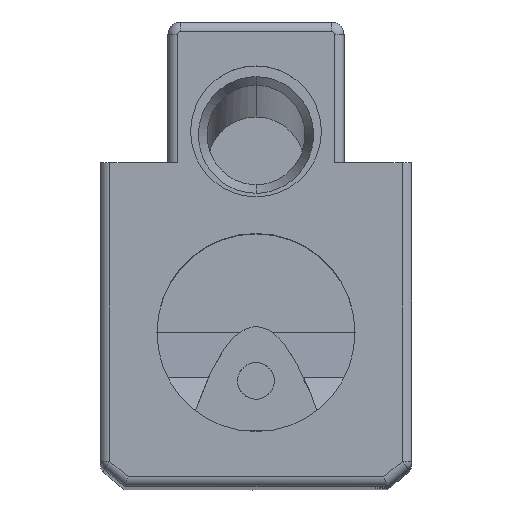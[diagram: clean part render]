
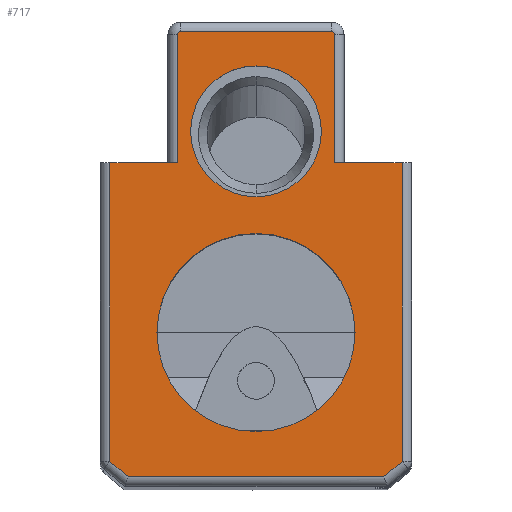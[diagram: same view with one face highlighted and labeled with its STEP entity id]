
A CAD part, top view. The second image highlights one B-rep face of the part: STEP entity #717.
In plain terms, the highlighted planar face has unit normal (0, 0, 1).
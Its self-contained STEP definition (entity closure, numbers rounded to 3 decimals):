
#1 = CARTESIAN_POINT ( 'NONE',  ( 8.1, -0.65, 0. ) ) ;
#50 = EDGE_LOOP ( 'NONE', ( #1934, #164 ) ) ;
#64 = VERTEX_POINT ( 'NONE', #5899 ) ;
#115 = AXIS2_PLACEMENT_3D ( 'NONE', #4630, #5019, #1920 ) ;
#150 = VERTEX_POINT ( 'NONE', #1952 ) ;
#164 = ORIENTED_EDGE ( 'NONE', *, *, #4117, .T. ) ;
#181 = DIRECTION ( 'NONE',  ( 1., 0., 0. ) ) ;
#234 = CARTESIAN_POINT ( 'NONE',  ( -6.2, 23.75, 0. ) ) ;
#284 = LINE ( 'NONE', #801, #3854 ) ;
#332 = EDGE_CURVE ( 'NONE', #5926, #869, #5600, .T. ) ;
#378 = ORIENTED_EDGE ( 'NONE', *, *, #2309, .F. ) ;
#432 = ORIENTED_EDGE ( 'NONE', *, *, #545, .T. ) ;
#531 = DIRECTION ( 'NONE',  ( 0., -1., 0. ) ) ;
#545 = EDGE_CURVE ( 'NONE', #1265, #2076, #2159, .T. ) ;
#591 = DIRECTION ( 'NONE',  ( 1., 0., 0. ) ) ;
#624 = CARTESIAN_POINT ( 'NONE',  ( 6.4, 23.75, 0. ) ) ;
#664 = CARTESIAN_POINT ( 'NONE',  ( 0., -0.65, 0. ) ) ;
#717 = ADVANCED_FACE ( 'NONE', ( #4224, #2316, #2632 ), #4130, .F. ) ;
#801 = CARTESIAN_POINT ( 'NONE',  ( -12.75, 13.25, 0. ) ) ;
#869 = VERTEX_POINT ( 'NONE', #1933 ) ;
#882 = VERTEX_POINT ( 'NONE', #3856 ) ;
#899 = DIRECTION ( 'NONE',  ( -0.766, -0.643, 0. ) ) ;
#955 = VERTEX_POINT ( 'NONE', #1 ) ;
#968 = ORIENTED_EDGE ( 'NONE', *, *, #332, .F. ) ;
#1054 = DIRECTION ( 'NONE',  ( -1., 0., 0. ) ) ;
#1068 = EDGE_CURVE ( 'NONE', #2082, #5395, #1801, .T. ) ;
#1101 = CARTESIAN_POINT ( 'NONE',  ( 5.35, 15.8, 0. ) ) ;
#1108 = DIRECTION ( 'NONE',  ( -1., 0., 0. ) ) ;
#1265 = VERTEX_POINT ( 'NONE', #624 ) ;
#1324 = ORIENTED_EDGE ( 'NONE', *, *, #4076, .T. ) ;
#1344 = EDGE_CURVE ( 'NONE', #5395, #2082, #5387, .T. ) ;
#1346 = EDGE_CURVE ( 'NONE', #150, #6261, #4244, .T. ) ;
#1401 = LINE ( 'NONE', #3632, #1552 ) ;
#1410 = AXIS2_PLACEMENT_3D ( 'NONE', #1907, #3327, #591 ) ;
#1411 = DIRECTION ( 'NONE',  ( 0., 0., -1. ) ) ;
#1472 = DIRECTION ( 'NONE',  ( 0., 0., -1. ) ) ;
#1508 = DIRECTION ( 'NONE',  ( 0., -1., 0. ) ) ;
#1552 = VECTOR ( 'NONE', #899, 1000. ) ;
#1577 = DIRECTION ( 'NONE',  ( -1., 0., 0. ) ) ;
#1602 = CARTESIAN_POINT ( 'NONE',  ( 11.95, -11.199, 0. ) ) ;
#1708 = AXIS2_PLACEMENT_3D ( 'NONE', #664, #1472, #1577 ) ;
#1737 = CARTESIAN_POINT ( 'NONE',  ( 10.459, -12.45, 0. ) ) ;
#1741 = ORIENTED_EDGE ( 'NONE', *, *, #3495, .T. ) ;
#1768 = AXIS2_PLACEMENT_3D ( 'NONE', #2861, #2649, #6206 ) ;
#1801 = CIRCLE ( 'NONE', #1410, 5.35 ) ;
#1907 = CARTESIAN_POINT ( 'NONE',  ( 0., 15.8, 0. ) ) ;
#1920 = DIRECTION ( 'NONE',  ( -1., 0., 0. ) ) ;
#1933 = CARTESIAN_POINT ( 'NONE',  ( -11.95, -11.199, 0. ) ) ;
#1934 = ORIENTED_EDGE ( 'NONE', *, *, #4635, .T. ) ;
#1951 = EDGE_CURVE ( 'NONE', #882, #150, #3329, .T. ) ;
#1952 = CARTESIAN_POINT ( 'NONE',  ( -6.4, 23.75, 0. ) ) ;
#1957 = EDGE_CURVE ( 'NONE', #869, #2942, #2252, .T. ) ;
#2065 = LINE ( 'NONE', #4367, #2939 ) ;
#2076 = VERTEX_POINT ( 'NONE', #4369 ) ;
#2082 = VERTEX_POINT ( 'NONE', #4871 ) ;
#2098 = VECTOR ( 'NONE', #4193, 1000. ) ;
#2135 = CARTESIAN_POINT ( 'NONE',  ( -10.459, -12.45, 0. ) ) ;
#2159 = CIRCLE ( 'NONE', #115, 0.2 ) ;
#2170 = CARTESIAN_POINT ( 'NONE',  ( -11.95, 13.25, 0. ) ) ;
#2176 = EDGE_LOOP ( 'NONE', ( #2567, #5139, #5936, #968, #3387, #4484, #378, #5836, #1324, #432, #1741, #4733 ) ) ;
#2223 = VERTEX_POINT ( 'NONE', #1602 ) ;
#2252 = LINE ( 'NONE', #5588, #5330 ) ;
#2261 = CARTESIAN_POINT ( 'NONE',  ( -6.2, 23.95, 0. ) ) ;
#2309 = EDGE_CURVE ( 'NONE', #4517, #2223, #3640, .T. ) ;
#2316 = FACE_OUTER_BOUND ( 'NONE', #2176, .T. ) ;
#2438 = VERTEX_POINT ( 'NONE', #1737 ) ;
#2483 = LINE ( 'NONE', #2261, #2767 ) ;
#2567 = ORIENTED_EDGE ( 'NONE', *, *, #1346, .T. ) ;
#2632 = FACE_BOUND ( 'NONE', #3348, .T. ) ;
#2649 = DIRECTION ( 'NONE',  ( 0., 0., 1. ) ) ;
#2767 = VECTOR ( 'NONE', #5596, 1000. ) ;
#2789 = VECTOR ( 'NONE', #1508, 1000. ) ;
#2861 = CARTESIAN_POINT ( 'NONE',  ( 0., 15.8, 0. ) ) ;
#2939 = VECTOR ( 'NONE', #4957, 1000. ) ;
#2942 = VERTEX_POINT ( 'NONE', #2170 ) ;
#3031 = EDGE_CURVE ( 'NONE', #2438, #5926, #2065, .T. ) ;
#3038 = DIRECTION ( 'NONE',  ( 0., 0., -1. ) ) ;
#3087 = DIRECTION ( 'NONE',  ( 0., 1., 0. ) ) ;
#3263 = CARTESIAN_POINT ( 'NONE',  ( -6.4, 13.25, 0. ) ) ;
#3327 = DIRECTION ( 'NONE',  ( 0., 0., 1. ) ) ;
#3329 = CIRCLE ( 'NONE', #5118, 0.2 ) ;
#3345 = CARTESIAN_POINT ( 'NONE',  ( 0., 0., 0. ) ) ;
#3348 = EDGE_LOOP ( 'NONE', ( #4192, #4687 ) ) ;
#3387 = ORIENTED_EDGE ( 'NONE', *, *, #3031, .F. ) ;
#3495 = EDGE_CURVE ( 'NONE', #2076, #882, #2483, .T. ) ;
#3632 = CARTESIAN_POINT ( 'NONE',  ( 11.95, -11.199, 0. ) ) ;
#3640 = LINE ( 'NONE', #3829, #2789 ) ;
#3713 = EDGE_CURVE ( 'NONE', #64, #4517, #4104, .T. ) ;
#3724 = DIRECTION ( 'NONE',  ( 0., 1., 0. ) ) ;
#3776 = DIRECTION ( 'NONE',  ( 0., 0., 1. ) ) ;
#3826 = DIRECTION ( 'NONE',  ( -1., 0., 0. ) ) ;
#3829 = CARTESIAN_POINT ( 'NONE',  ( 11.95, 0., 0. ) ) ;
#3853 = VECTOR ( 'NONE', #5815, 1000. ) ;
#3854 = VECTOR ( 'NONE', #181, 1000. ) ;
#3856 = CARTESIAN_POINT ( 'NONE',  ( -6.2, 23.95, 0. ) ) ;
#3871 = VECTOR ( 'NONE', #3724, 1000. ) ;
#4006 = AXIS2_PLACEMENT_3D ( 'NONE', #3345, #1411, #1108 ) ;
#4053 = CARTESIAN_POINT ( 'NONE',  ( -6.4, 13.25, 0. ) ) ;
#4069 = EDGE_CURVE ( 'NONE', #2223, #2438, #1401, .T. ) ;
#4076 = EDGE_CURVE ( 'NONE', #64, #1265, #5002, .T. ) ;
#4104 = LINE ( 'NONE', #5088, #2098 ) ;
#4117 = EDGE_CURVE ( 'NONE', #6094, #955, #5649, .T. ) ;
#4129 = CIRCLE ( 'NONE', #1708, 8.1 ) ;
#4130 = PLANE ( 'NONE',  #4006 ) ;
#4192 = ORIENTED_EDGE ( 'NONE', *, *, #1344, .F. ) ;
#4193 = DIRECTION ( 'NONE',  ( 1., 0., 0. ) ) ;
#4224 = FACE_BOUND ( 'NONE', #50, .T. ) ;
#4244 = LINE ( 'NONE', #3263, #4657 ) ;
#4249 = AXIS2_PLACEMENT_3D ( 'NONE', #5742, #3038, #3826 ) ;
#4297 = CARTESIAN_POINT ( 'NONE',  ( 11.95, 13.25, 0. ) ) ;
#4367 = CARTESIAN_POINT ( 'NONE',  ( 0., -12.45, 0. ) ) ;
#4369 = CARTESIAN_POINT ( 'NONE',  ( 6.2, 23.95, 0. ) ) ;
#4484 = ORIENTED_EDGE ( 'NONE', *, *, #4069, .F. ) ;
#4517 = VERTEX_POINT ( 'NONE', #4297 ) ;
#4527 = CARTESIAN_POINT ( 'NONE',  ( -8.1, -0.65, 0. ) ) ;
#4630 = CARTESIAN_POINT ( 'NONE',  ( 6.2, 23.75, 0. ) ) ;
#4635 = EDGE_CURVE ( 'NONE', #955, #6094, #4129, .T. ) ;
#4657 = VECTOR ( 'NONE', #531, 1000. ) ;
#4687 = ORIENTED_EDGE ( 'NONE', *, *, #1068, .F. ) ;
#4733 = ORIENTED_EDGE ( 'NONE', *, *, #1951, .T. ) ;
#4751 = EDGE_CURVE ( 'NONE', #2942, #6261, #284, .T. ) ;
#4871 = CARTESIAN_POINT ( 'NONE',  ( -5.35, 15.8, 0. ) ) ;
#4957 = DIRECTION ( 'NONE',  ( -1., 0., 0. ) ) ;
#5002 = LINE ( 'NONE', #5325, #3871 ) ;
#5019 = DIRECTION ( 'NONE',  ( 0., 0., 1. ) ) ;
#5088 = CARTESIAN_POINT ( 'NONE',  ( -12.75, 13.25, 0. ) ) ;
#5118 = AXIS2_PLACEMENT_3D ( 'NONE', #234, #3776, #1054 ) ;
#5139 = ORIENTED_EDGE ( 'NONE', *, *, #4751, .F. ) ;
#5325 = CARTESIAN_POINT ( 'NONE',  ( 6.4, 0., 0. ) ) ;
#5330 = VECTOR ( 'NONE', #3087, 1000. ) ;
#5387 = CIRCLE ( 'NONE', #1768, 5.35 ) ;
#5395 = VERTEX_POINT ( 'NONE', #1101 ) ;
#5588 = CARTESIAN_POINT ( 'NONE',  ( -11.95, 0., 0. ) ) ;
#5596 = DIRECTION ( 'NONE',  ( -1., 0., 0. ) ) ;
#5600 = LINE ( 'NONE', #6144, #3853 ) ;
#5649 = CIRCLE ( 'NONE', #4249, 8.1 ) ;
#5742 = CARTESIAN_POINT ( 'NONE',  ( 0., -0.65, 0. ) ) ;
#5815 = DIRECTION ( 'NONE',  ( -0.766, 0.643, 0. ) ) ;
#5836 = ORIENTED_EDGE ( 'NONE', *, *, #3713, .F. ) ;
#5899 = CARTESIAN_POINT ( 'NONE',  ( 6.4, 13.25, 0. ) ) ;
#5926 = VERTEX_POINT ( 'NONE', #2135 ) ;
#5936 = ORIENTED_EDGE ( 'NONE', *, *, #1957, .F. ) ;
#6094 = VERTEX_POINT ( 'NONE', #4527 ) ;
#6144 = CARTESIAN_POINT ( 'NONE',  ( -10.459, -12.45, 0. ) ) ;
#6206 = DIRECTION ( 'NONE',  ( 1., 0., 0. ) ) ;
#6261 = VERTEX_POINT ( 'NONE', #4053 ) ;
